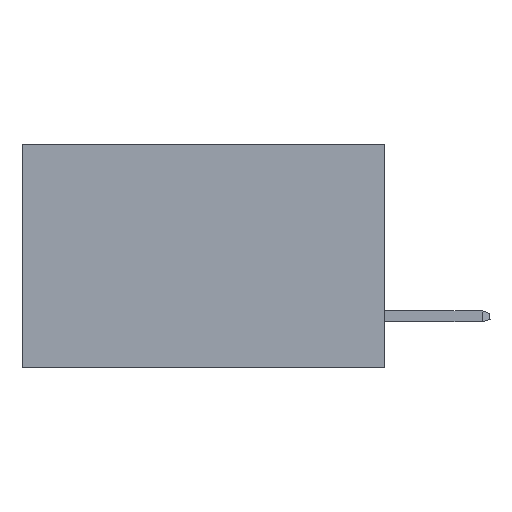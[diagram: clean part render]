
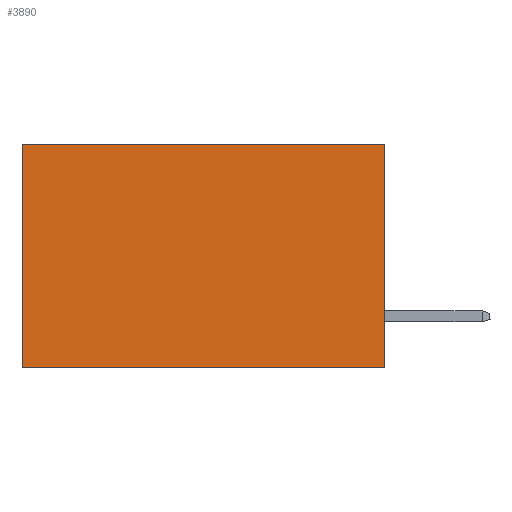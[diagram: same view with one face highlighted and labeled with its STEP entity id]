
A CAD part, left-side view. The second image highlights one B-rep face of the part: STEP entity #3890.
In plain terms, the highlighted planar face has unit normal (-1, 0, 0).
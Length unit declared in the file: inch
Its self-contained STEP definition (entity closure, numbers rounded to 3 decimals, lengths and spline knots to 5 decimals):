
#327 = DIRECTION ( 'NONE',  ( 1., 0., 0. ) ) ;
#585 = ORIENTED_EDGE ( 'NONE', *, *, #788, .F. ) ;
#617 = DIRECTION ( 'NONE',  ( 0., 0., -1. ) ) ;
#788 = EDGE_CURVE ( 'NONE', #8565, #16426, #17982, .T. ) ;
#1199 = CARTESIAN_POINT ( 'NONE',  ( 0.298, 0., 0. ) ) ;
#2106 = ORIENTED_EDGE ( 'NONE', *, *, #11515, .T. ) ;
#2180 = ORIENTED_EDGE ( 'NONE', *, *, #11174, .F. ) ;
#2478 = AXIS2_PLACEMENT_3D ( 'NONE', #11444, #327, #16964 ) ;
#2529 = DIRECTION ( 'NONE',  ( 0., 1., 0. ) ) ;
#3890 = ADVANCED_FACE ( 'NONE', ( #4170 ), #15669, .F. ) ;
#4170 = FACE_OUTER_BOUND ( 'NONE', #4740, .T. ) ;
#4740 = EDGE_LOOP ( 'NONE', ( #2106, #585, #2180, #11321 ) ) ;
#5567 = VERTEX_POINT ( 'NONE', #10147 ) ;
#8006 = DIRECTION ( 'NONE',  ( 0., 1., 0. ) ) ;
#8222 = DIRECTION ( 'NONE',  ( 0., 0., -1. ) ) ;
#8365 = VECTOR ( 'NONE', #8006, 39.37008 ) ;
#8565 = VERTEX_POINT ( 'NONE', #10464 ) ;
#9639 = CARTESIAN_POINT ( 'NONE',  ( 0.298, 0.6, 0. ) ) ;
#10147 = CARTESIAN_POINT ( 'NONE',  ( 0.298, 0.6, 0. ) ) ;
#10464 = CARTESIAN_POINT ( 'NONE',  ( 0.298, 0., -0.37 ) ) ;
#11073 = EDGE_CURVE ( 'NONE', #13979, #5567, #17995, .T. ) ;
#11174 = EDGE_CURVE ( 'NONE', #13979, #8565, #15997, .T. ) ;
#11321 = ORIENTED_EDGE ( 'NONE', *, *, #11073, .T. ) ;
#11444 = CARTESIAN_POINT ( 'NONE',  ( 0.298, 0., 0. ) ) ;
#11515 = EDGE_CURVE ( 'NONE', #5567, #16426, #17317, .T. ) ;
#13738 = CARTESIAN_POINT ( 'NONE',  ( 0.298, 0., -0.37 ) ) ;
#13979 = VERTEX_POINT ( 'NONE', #17684 ) ;
#14286 = CARTESIAN_POINT ( 'NONE',  ( 0.298, 0., 0. ) ) ;
#14689 = VECTOR ( 'NONE', #617, 39.37008 ) ;
#15124 = VECTOR ( 'NONE', #8222, 39.37008 ) ;
#15169 = CARTESIAN_POINT ( 'NONE',  ( 0.298, 0.6, -0.37 ) ) ;
#15669 = PLANE ( 'NONE',  #2478 ) ;
#15997 = LINE ( 'NONE', #14286, #14689 ) ;
#16426 = VERTEX_POINT ( 'NONE', #15169 ) ;
#16964 = DIRECTION ( 'NONE',  ( 0., 0., -1. ) ) ;
#17317 = LINE ( 'NONE', #9639, #15124 ) ;
#17554 = VECTOR ( 'NONE', #2529, 39.37008 ) ;
#17684 = CARTESIAN_POINT ( 'NONE',  ( 0.298, 0., 0. ) ) ;
#17982 = LINE ( 'NONE', #13738, #8365 ) ;
#17995 = LINE ( 'NONE', #1199, #17554 ) ;
